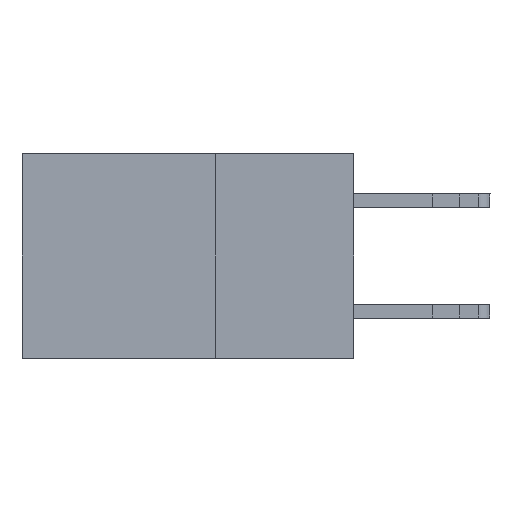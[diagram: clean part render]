
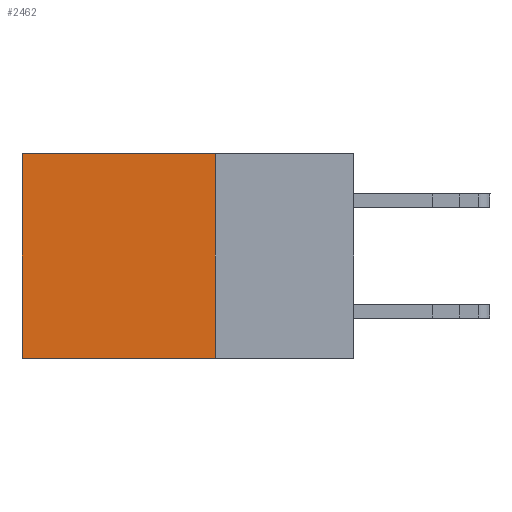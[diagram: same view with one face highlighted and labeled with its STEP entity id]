
A CAD part, left-side view. The second image highlights one B-rep face of the part: STEP entity #2462.
In plain terms, the highlighted planar face has unit normal (-1, 0, 0).
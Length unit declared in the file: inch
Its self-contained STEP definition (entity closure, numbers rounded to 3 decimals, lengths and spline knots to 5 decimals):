
#1411 = AXIS2_PLACEMENT_3D ( 'NONE', #26562, #13267, #18580 ) ;
#2094 = EDGE_LOOP ( 'NONE', ( #13537, #30739, #11843, #16318 ) ) ;
#2462 = ADVANCED_FACE ( 'NONE', ( #11347 ), #21341, .F. ) ;
#2962 = EDGE_CURVE ( 'NONE', #23552, #4742, #6352, .T. ) ;
#4083 = DIRECTION ( 'NONE',  ( 0., 0., -1. ) ) ;
#4344 = CARTESIAN_POINT ( 'NONE',  ( 0.2875, 0.6, 0. ) ) ;
#4742 = VERTEX_POINT ( 'NONE', #31811 ) ;
#6305 = LINE ( 'NONE', #7487, #26599 ) ;
#6352 = LINE ( 'NONE', #23734, #26645 ) ;
#7487 = CARTESIAN_POINT ( 'NONE',  ( 0.2875, 0.25, 0. ) ) ;
#10021 = CARTESIAN_POINT ( 'NONE',  ( 0.2875, 0.6, -0.37 ) ) ;
#10988 = VERTEX_POINT ( 'NONE', #10021 ) ;
#11347 = FACE_OUTER_BOUND ( 'NONE', #2094, .T. ) ;
#11843 = ORIENTED_EDGE ( 'NONE', *, *, #2962, .F. ) ;
#12054 = LINE ( 'NONE', #20029, #14124 ) ;
#12314 = DIRECTION ( 'NONE',  ( 0., 1., 0. ) ) ;
#13267 = DIRECTION ( 'NONE',  ( 1., 0., 0. ) ) ;
#13537 = ORIENTED_EDGE ( 'NONE', *, *, #13896, .T. ) ;
#13896 = EDGE_CURVE ( 'NONE', #19987, #10988, #27699, .T. ) ;
#14124 = VECTOR ( 'NONE', #12314, 39.37008 ) ;
#16318 = ORIENTED_EDGE ( 'NONE', *, *, #20809, .T. ) ;
#17153 = CARTESIAN_POINT ( 'NONE',  ( 0.2875, 0.6, 0. ) ) ;
#18580 = DIRECTION ( 'NONE',  ( 0., 0., -1. ) ) ;
#19987 = VERTEX_POINT ( 'NONE', #4344 ) ;
#20029 = CARTESIAN_POINT ( 'NONE',  ( 0.2875, 0.25, -0.37 ) ) ;
#20809 = EDGE_CURVE ( 'NONE', #23552, #19987, #6305, .T. ) ;
#21259 = EDGE_CURVE ( 'NONE', #4742, #10988, #12054, .T. ) ;
#21341 = PLANE ( 'NONE',  #1411 ) ;
#22841 = DIRECTION ( 'NONE',  ( 0., 1., 0. ) ) ;
#23552 = VERTEX_POINT ( 'NONE', #29388 ) ;
#23734 = CARTESIAN_POINT ( 'NONE',  ( 0.2875, 0.25, 0. ) ) ;
#26518 = DIRECTION ( 'NONE',  ( 0., 0., -1. ) ) ;
#26562 = CARTESIAN_POINT ( 'NONE',  ( 0.2875, 0.25, 0. ) ) ;
#26599 = VECTOR ( 'NONE', #22841, 39.37008 ) ;
#26645 = VECTOR ( 'NONE', #26518, 39.37008 ) ;
#26901 = VECTOR ( 'NONE', #4083, 39.37008 ) ;
#27699 = LINE ( 'NONE', #17153, #26901 ) ;
#29388 = CARTESIAN_POINT ( 'NONE',  ( 0.2875, 0.25, 0. ) ) ;
#30739 = ORIENTED_EDGE ( 'NONE', *, *, #21259, .F. ) ;
#31811 = CARTESIAN_POINT ( 'NONE',  ( 0.2875, 0.25, -0.37 ) ) ;
